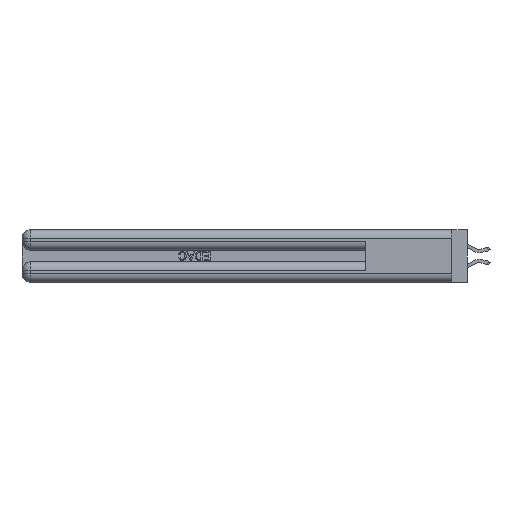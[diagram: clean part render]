
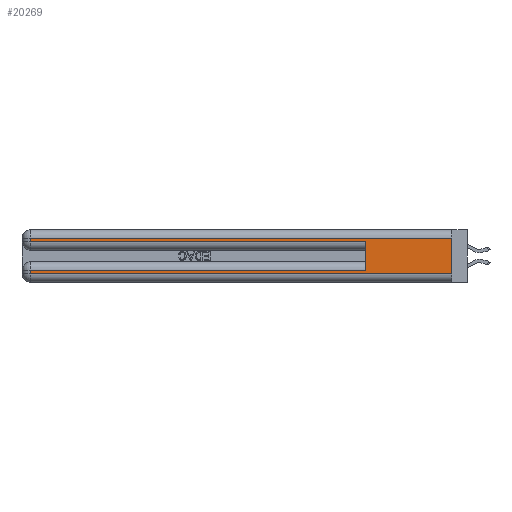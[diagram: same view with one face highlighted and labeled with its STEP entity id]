
A CAD part, left-side view. The second image highlights one B-rep face of the part: STEP entity #20269.
In plain terms, the highlighted planar face has unit normal (-1, 0, 0).
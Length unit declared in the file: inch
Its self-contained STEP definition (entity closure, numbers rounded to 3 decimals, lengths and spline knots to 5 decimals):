
#529 = DIRECTION ( 'NONE',  ( 0., -1., 0. ) ) ;
#1032 = VERTEX_POINT ( 'NONE', #11321 ) ;
#1424 = CARTESIAN_POINT ( 'NONE',  ( 0., 0., 0.285 ) ) ;
#1583 = CARTESIAN_POINT ( 'NONE',  ( 0., 0., 0.085 ) ) ;
#2993 = VECTOR ( 'NONE', #23736, 39.37008 ) ;
#3997 = EDGE_CURVE ( 'NONE', #16902, #5636, #43032, .T. ) ;
#4109 = VECTOR ( 'NONE', #529, 39.37008 ) ;
#4191 = LINE ( 'NONE', #18885, #15678 ) ;
#5535 = EDGE_CURVE ( 'NONE', #16902, #42267, #25495, .T. ) ;
#5536 = CARTESIAN_POINT ( 'NONE',  ( 0., 2.94, 0.06 ) ) ;
#5636 = VERTEX_POINT ( 'NONE', #33971 ) ;
#7879 = VECTOR ( 'NONE', #9247, 39.37008 ) ;
#9247 = DIRECTION ( 'NONE',  ( 0., 1., 0. ) ) ;
#10876 = ORIENTED_EDGE ( 'NONE', *, *, #30773, .T. ) ;
#11152 = ORIENTED_EDGE ( 'NONE', *, *, #27874, .F. ) ;
#11249 = VERTEX_POINT ( 'NONE', #25547 ) ;
#11321 = CARTESIAN_POINT ( 'NONE',  ( 0., 0.6, 0.285 ) ) ;
#11819 = VECTOR ( 'NONE', #33797, 39.37008 ) ;
#12917 = CARTESIAN_POINT ( 'NONE',  ( 0., 0., 0.31 ) ) ;
#13754 = ORIENTED_EDGE ( 'NONE', *, *, #24120, .T. ) ;
#13914 = LINE ( 'NONE', #1583, #7879 ) ;
#13927 = CARTESIAN_POINT ( 'NONE',  ( 0., 2.94, 0.37 ) ) ;
#15010 = LINE ( 'NONE', #25215, #4109 ) ;
#15402 = LINE ( 'NONE', #17167, #16517 ) ;
#15678 = VECTOR ( 'NONE', #39864, 39.37008 ) ;
#16517 = VECTOR ( 'NONE', #44566, 39.37008 ) ;
#16774 = CARTESIAN_POINT ( 'NONE',  ( 0., 0., 0.37 ) ) ;
#16902 = VERTEX_POINT ( 'NONE', #18889 ) ;
#17167 = CARTESIAN_POINT ( 'NONE',  ( 0., 0.6, 0.145 ) ) ;
#17627 = DIRECTION ( 'NONE',  ( 0., 1., 0. ) ) ;
#18885 = CARTESIAN_POINT ( 'NONE',  ( 0., 2.94, 0.37 ) ) ;
#18889 = CARTESIAN_POINT ( 'NONE',  ( 0., 0., 0.31 ) ) ;
#19436 = ORIENTED_EDGE ( 'NONE', *, *, #33645, .T. ) ;
#20024 = ORIENTED_EDGE ( 'NONE', *, *, #5535, .T. ) ;
#20143 = EDGE_LOOP ( 'NONE', ( #25338, #20024, #19436, #13754, #11152, #27445, #10876, #32864 ) ) ;
#20269 = ADVANCED_FACE ( 'NONE', ( #28248 ), #44038, .F. ) ;
#23055 = CARTESIAN_POINT ( 'NONE',  ( 0., 0.6, 0.085 ) ) ;
#23378 = DIRECTION ( 'NONE',  ( 0., 0., -1. ) ) ;
#23736 = DIRECTION ( 'NONE',  ( 0., 0., -1. ) ) ;
#24120 = EDGE_CURVE ( 'NONE', #11249, #1032, #40734, .T. ) ;
#25215 = CARTESIAN_POINT ( 'NONE',  ( 0., 0., 0.06 ) ) ;
#25338 = ORIENTED_EDGE ( 'NONE', *, *, #3997, .F. ) ;
#25495 = LINE ( 'NONE', #12917, #27154 ) ;
#25547 = CARTESIAN_POINT ( 'NONE',  ( 0., 2.94, 0.285 ) ) ;
#26995 = DIRECTION ( 'NONE',  ( 1., 0., 0. ) ) ;
#27154 = VECTOR ( 'NONE', #17627, 39.37008 ) ;
#27445 = ORIENTED_EDGE ( 'NONE', *, *, #40850, .T. ) ;
#27874 = EDGE_CURVE ( 'NONE', #38761, #1032, #15402, .T. ) ;
#28248 = FACE_OUTER_BOUND ( 'NONE', #20143, .T. ) ;
#30181 = LINE ( 'NONE', #13927, #2993 ) ;
#30773 = EDGE_CURVE ( 'NONE', #42900, #31503, #4191, .T. ) ;
#31503 = VERTEX_POINT ( 'NONE', #5536 ) ;
#32379 = EDGE_CURVE ( 'NONE', #31503, #5636, #15010, .T. ) ;
#32864 = ORIENTED_EDGE ( 'NONE', *, *, #32379, .T. ) ;
#33645 = EDGE_CURVE ( 'NONE', #42267, #11249, #30181, .T. ) ;
#33797 = DIRECTION ( 'NONE',  ( 0., -1., 0. ) ) ;
#33971 = CARTESIAN_POINT ( 'NONE',  ( 0., 0., 0.06 ) ) ;
#35389 = VECTOR ( 'NONE', #41410, 39.37008 ) ;
#37399 = AXIS2_PLACEMENT_3D ( 'NONE', #44192, #26995, #23378 ) ;
#38404 = CARTESIAN_POINT ( 'NONE',  ( 0., 2.94, 0.31 ) ) ;
#38761 = VERTEX_POINT ( 'NONE', #23055 ) ;
#39864 = DIRECTION ( 'NONE',  ( 0., 0., -1. ) ) ;
#40734 = LINE ( 'NONE', #1424, #11819 ) ;
#40850 = EDGE_CURVE ( 'NONE', #38761, #42900, #13914, .T. ) ;
#41410 = DIRECTION ( 'NONE',  ( 0., 0., -1. ) ) ;
#42168 = CARTESIAN_POINT ( 'NONE',  ( 0., 2.94, 0.085 ) ) ;
#42267 = VERTEX_POINT ( 'NONE', #38404 ) ;
#42900 = VERTEX_POINT ( 'NONE', #42168 ) ;
#43032 = LINE ( 'NONE', #16774, #35389 ) ;
#44038 = PLANE ( 'NONE',  #37399 ) ;
#44192 = CARTESIAN_POINT ( 'NONE',  ( 0., 0., 0.37 ) ) ;
#44566 = DIRECTION ( 'NONE',  ( 0., 0., 1. ) ) ;
